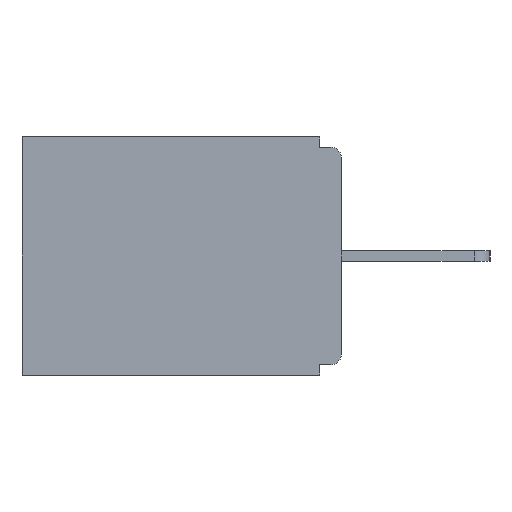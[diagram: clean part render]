
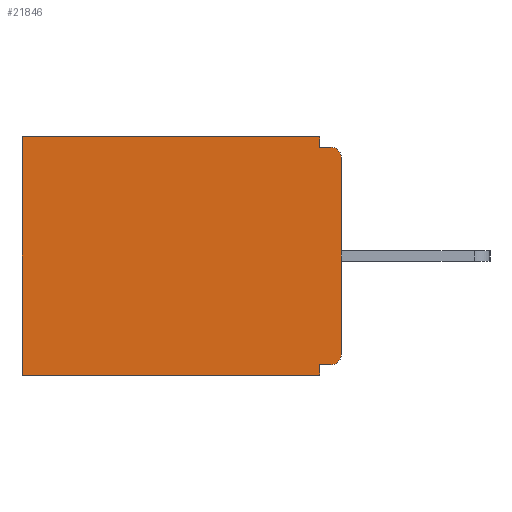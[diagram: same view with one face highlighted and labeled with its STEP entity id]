
A CAD part, left-side view. The second image highlights one B-rep face of the part: STEP entity #21846.
In plain terms, the highlighted planar face has unit normal (-1, 0, 0).
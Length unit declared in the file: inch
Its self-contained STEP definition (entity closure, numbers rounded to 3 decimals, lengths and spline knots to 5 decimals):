
#707 = VECTOR ( 'NONE', #5480, 39.37008 ) ;
#920 = CARTESIAN_POINT ( 'NONE',  ( 0.298, 0.031, -0.343 ) ) ;
#988 = EDGE_CURVE ( 'NONE', #15541, #21546, #10243, .T. ) ;
#1017 = VERTEX_POINT ( 'NONE', #13460 ) ;
#1121 = VERTEX_POINT ( 'NONE', #23494 ) ;
#1529 = VECTOR ( 'NONE', #21109, 39.37008 ) ;
#2030 = EDGE_CURVE ( 'NONE', #18419, #17198, #21994, .T. ) ;
#2210 = ORIENTED_EDGE ( 'NONE', *, *, #20839, .F. ) ;
#2653 = EDGE_CURVE ( 'NONE', #18419, #1121, #4662, .T. ) ;
#2811 = AXIS2_PLACEMENT_3D ( 'NONE', #11688, #19073, #15493 ) ;
#3010 = ORIENTED_EDGE ( 'NONE', *, *, #7208, .F. ) ;
#3044 = AXIS2_PLACEMENT_3D ( 'NONE', #19079, #12046, #15364 ) ;
#3198 = LINE ( 'NONE', #920, #17696 ) ;
#3487 = EDGE_CURVE ( 'NONE', #21546, #6071, #10406, .T. ) ;
#4053 = EDGE_CURVE ( 'NONE', #15720, #6071, #15963, .T. ) ;
#4414 = ORIENTED_EDGE ( 'NONE', *, *, #988, .T. ) ;
#4416 = PLANE ( 'NONE',  #3044 ) ;
#4662 = CIRCLE ( 'NONE', #10354, 0.015 ) ;
#4728 = ORIENTED_EDGE ( 'NONE', *, *, #4053, .F. ) ;
#4870 = CARTESIAN_POINT ( 'NONE',  ( 0.298, 0.031, -0.343 ) ) ;
#5480 = DIRECTION ( 'NONE',  ( 0., 0., -1. ) ) ;
#6071 = VERTEX_POINT ( 'NONE', #12835 ) ;
#6073 = EDGE_LOOP ( 'NONE', ( #20007, #6430, #3010, #4414, #16417, #4728, #2210, #14386, #6687, #10598 ) ) ;
#6191 = FACE_OUTER_BOUND ( 'NONE', #6073, .T. ) ;
#6430 = ORIENTED_EDGE ( 'NONE', *, *, #20824, .F. ) ;
#6548 = VERTEX_POINT ( 'NONE', #18837 ) ;
#6687 = ORIENTED_EDGE ( 'NONE', *, *, #12386, .T. ) ;
#6947 = DIRECTION ( 'NONE',  ( 0., 1., 0. ) ) ;
#7208 = EDGE_CURVE ( 'NONE', #15541, #20326, #3198, .T. ) ;
#7362 = CIRCLE ( 'NONE', #2811, 0.015 ) ;
#7764 = DIRECTION ( 'NONE',  ( 0., 0., -1. ) ) ;
#8090 = DIRECTION ( 'NONE',  ( 0., 0., -1. ) ) ;
#8889 = CARTESIAN_POINT ( 'NONE',  ( 0.298, 0., -0.313 ) ) ;
#9652 = DIRECTION ( 'NONE',  ( -1., 0., 0. ) ) ;
#10243 = LINE ( 'NONE', #13704, #1529 ) ;
#10282 = CARTESIAN_POINT ( 'NONE',  ( 0.298, 0.031, -0.015 ) ) ;
#10354 = AXIS2_PLACEMENT_3D ( 'NONE', #11460, #9652, #8090 ) ;
#10406 = LINE ( 'NONE', #10654, #15856 ) ;
#10598 = ORIENTED_EDGE ( 'NONE', *, *, #2030, .F. ) ;
#10654 = CARTESIAN_POINT ( 'NONE',  ( 0.298, 0.46, 0. ) ) ;
#10668 = VECTOR ( 'NONE', #7764, 39.37008 ) ;
#10993 = VECTOR ( 'NONE', #20164, 39.37008 ) ;
#11347 = VECTOR ( 'NONE', #6947, 39.37008 ) ;
#11460 = CARTESIAN_POINT ( 'NONE',  ( 0.298, 0.015, -0.03 ) ) ;
#11688 = CARTESIAN_POINT ( 'NONE',  ( 0.298, 0.015, -0.313 ) ) ;
#12046 = DIRECTION ( 'NONE',  ( 1., 0., 0. ) ) ;
#12330 = LINE ( 'NONE', #19608, #11347 ) ;
#12386 = EDGE_CURVE ( 'NONE', #1017, #17198, #7362, .T. ) ;
#12419 = LINE ( 'NONE', #14535, #10993 ) ;
#12835 = CARTESIAN_POINT ( 'NONE',  ( 0.298, 0.46, -0.343 ) ) ;
#13460 = CARTESIAN_POINT ( 'NONE',  ( 0.298, 0.015, -0.328 ) ) ;
#13704 = CARTESIAN_POINT ( 'NONE',  ( 0.298, 0., 0. ) ) ;
#13923 = CARTESIAN_POINT ( 'NONE',  ( 0.298, 0., -0.343 ) ) ;
#14386 = ORIENTED_EDGE ( 'NONE', *, *, #20366, .F. ) ;
#14535 = CARTESIAN_POINT ( 'NONE',  ( 0.298, 0., -0.015 ) ) ;
#15364 = DIRECTION ( 'NONE',  ( 0., 0., -1. ) ) ;
#15493 = DIRECTION ( 'NONE',  ( 0., 0., -1. ) ) ;
#15541 = VERTEX_POINT ( 'NONE', #16537 ) ;
#15720 = VERTEX_POINT ( 'NONE', #4870 ) ;
#15856 = VECTOR ( 'NONE', #23303, 39.37008 ) ;
#15963 = LINE ( 'NONE', #13923, #19293 ) ;
#16417 = ORIENTED_EDGE ( 'NONE', *, *, #3487, .T. ) ;
#16537 = CARTESIAN_POINT ( 'NONE',  ( 0.298, 0.031, 0. ) ) ;
#16619 = CARTESIAN_POINT ( 'NONE',  ( 0.298, 0., 0. ) ) ;
#17198 = VERTEX_POINT ( 'NONE', #8889 ) ;
#17696 = VECTOR ( 'NONE', #21450, 39.37008 ) ;
#17967 = CARTESIAN_POINT ( 'NONE',  ( 0.298, 0., -0.03 ) ) ;
#18419 = VERTEX_POINT ( 'NONE', #17967 ) ;
#18837 = CARTESIAN_POINT ( 'NONE',  ( 0.298, 0.031, -0.328 ) ) ;
#19073 = DIRECTION ( 'NONE',  ( -1., 0., 0. ) ) ;
#19079 = CARTESIAN_POINT ( 'NONE',  ( 0.298, 0., 0. ) ) ;
#19293 = VECTOR ( 'NONE', #21213, 39.37008 ) ;
#19481 = CARTESIAN_POINT ( 'NONE',  ( 0.298, 0.46, 0. ) ) ;
#19608 = CARTESIAN_POINT ( 'NONE',  ( 0.298, 0., -0.328 ) ) ;
#20007 = ORIENTED_EDGE ( 'NONE', *, *, #2653, .T. ) ;
#20164 = DIRECTION ( 'NONE',  ( 0., -1., 0. ) ) ;
#20326 = VERTEX_POINT ( 'NONE', #10282 ) ;
#20366 = EDGE_CURVE ( 'NONE', #1017, #6548, #12330, .T. ) ;
#20824 = EDGE_CURVE ( 'NONE', #20326, #1121, #12419, .T. ) ;
#20839 = EDGE_CURVE ( 'NONE', #6548, #15720, #21608, .T. ) ;
#21109 = DIRECTION ( 'NONE',  ( 0., 1., 0. ) ) ;
#21213 = DIRECTION ( 'NONE',  ( 0., 1., 0. ) ) ;
#21450 = DIRECTION ( 'NONE',  ( 0., 0., -1. ) ) ;
#21546 = VERTEX_POINT ( 'NONE', #19481 ) ;
#21608 = LINE ( 'NONE', #21718, #707 ) ;
#21718 = CARTESIAN_POINT ( 'NONE',  ( 0.298, 0.031, -0.343 ) ) ;
#21846 = ADVANCED_FACE ( 'NONE', ( #6191 ), #4416, .F. ) ;
#21994 = LINE ( 'NONE', #16619, #10668 ) ;
#23303 = DIRECTION ( 'NONE',  ( 0., 0., -1. ) ) ;
#23494 = CARTESIAN_POINT ( 'NONE',  ( 0.298, 0.015, -0.015 ) ) ;
